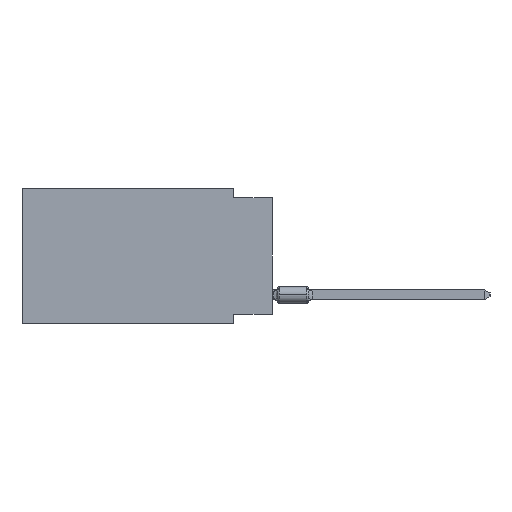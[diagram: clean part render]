
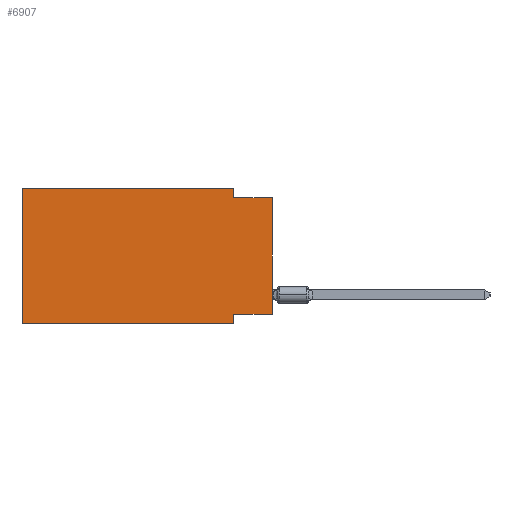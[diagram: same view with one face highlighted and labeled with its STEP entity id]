
A CAD part, left-side view. The second image highlights one B-rep face of the part: STEP entity #6907.
In plain terms, the highlighted planar face has unit normal (-1, 0, 0).
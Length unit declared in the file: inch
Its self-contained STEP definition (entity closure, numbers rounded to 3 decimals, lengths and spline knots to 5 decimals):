
#610 = VECTOR ( 'NONE', #41238, 39.37008 ) ;
#1041 = VECTOR ( 'NONE', #1689, 39.37008 ) ;
#1187 = VECTOR ( 'NONE', #8489, 39.37008 ) ;
#1689 = DIRECTION ( 'NONE',  ( 0., -1., 0. ) ) ;
#2277 = CARTESIAN_POINT ( 'NONE',  ( 0., 0.1, 0. ) ) ;
#2624 = CARTESIAN_POINT ( 'NONE',  ( 0., 0.1, -0.35 ) ) ;
#3584 = ORIENTED_EDGE ( 'NONE', *, *, #57239, .F. ) ;
#3718 = LINE ( 'NONE', #58554, #53860 ) ;
#4580 = VECTOR ( 'NONE', #31897, 39.37008 ) ;
#5265 = AXIS2_PLACEMENT_3D ( 'NONE', #47965, #54159, #21630 ) ;
#6539 = VECTOR ( 'NONE', #70454, 39.37008 ) ;
#6708 = EDGE_LOOP ( 'NONE', ( #24341, #24672, #17995, #44795, #29395, #54396, #44613, #3584 ) ) ;
#6907 = ADVANCED_FACE ( 'NONE', ( #42833 ), #60346, .F. ) ;
#7914 = VERTEX_POINT ( 'NONE', #2277 ) ;
#8489 = DIRECTION ( 'NONE',  ( 0., 0., -1. ) ) ;
#9325 = CARTESIAN_POINT ( 'NONE',  ( 0., 0.645, -0.35 ) ) ;
#17995 = ORIENTED_EDGE ( 'NONE', *, *, #40372, .F. ) ;
#19699 = LINE ( 'NONE', #24087, #38168 ) ;
#21630 = DIRECTION ( 'NONE',  ( 0., 0., -1. ) ) ;
#22252 = CARTESIAN_POINT ( 'NONE',  ( 0., 0.1, -0.325 ) ) ;
#22635 = DIRECTION ( 'NONE',  ( 0., 0., 1. ) ) ;
#22659 = VECTOR ( 'NONE', #22635, 39.37008 ) ;
#24087 = CARTESIAN_POINT ( 'NONE',  ( 0., 0.1, 0. ) ) ;
#24341 = ORIENTED_EDGE ( 'NONE', *, *, #68947, .T. ) ;
#24672 = ORIENTED_EDGE ( 'NONE', *, *, #59689, .F. ) ;
#24798 = CARTESIAN_POINT ( 'NONE',  ( 0., 0., 0. ) ) ;
#27245 = CARTESIAN_POINT ( 'NONE',  ( 0., 0., -0.025 ) ) ;
#29395 = ORIENTED_EDGE ( 'NONE', *, *, #30572, .F. ) ;
#30572 = EDGE_CURVE ( 'NONE', #43795, #34053, #61739, .T. ) ;
#30581 = LINE ( 'NONE', #52861, #1041 ) ;
#31017 = CARTESIAN_POINT ( 'NONE',  ( 0., 0., -0.325 ) ) ;
#31897 = DIRECTION ( 'NONE',  ( 0., -1., 0. ) ) ;
#33241 = CARTESIAN_POINT ( 'NONE',  ( 0., 0.645, 0. ) ) ;
#34053 = VERTEX_POINT ( 'NONE', #42239 ) ;
#34160 = VERTEX_POINT ( 'NONE', #27245 ) ;
#37383 = LINE ( 'NONE', #59661, #4580 ) ;
#38168 = VECTOR ( 'NONE', #47091, 39.37008 ) ;
#38562 = VERTEX_POINT ( 'NONE', #22252 ) ;
#40372 = EDGE_CURVE ( 'NONE', #7914, #53536, #19699, .T. ) ;
#41238 = DIRECTION ( 'NONE',  ( 0., 0., 1. ) ) ;
#42239 = CARTESIAN_POINT ( 'NONE',  ( 0., 0.645, 0. ) ) ;
#42833 = FACE_OUTER_BOUND ( 'NONE', #6708, .T. ) ;
#43795 = VERTEX_POINT ( 'NONE', #9325 ) ;
#44613 = ORIENTED_EDGE ( 'NONE', *, *, #59525, .F. ) ;
#44795 = ORIENTED_EDGE ( 'NONE', *, *, #47844, .F. ) ;
#46733 = LINE ( 'NONE', #24798, #610 ) ;
#47091 = DIRECTION ( 'NONE',  ( 0., 0., -1. ) ) ;
#47842 = CARTESIAN_POINT ( 'NONE',  ( 0., 0., -0.325 ) ) ;
#47844 = EDGE_CURVE ( 'NONE', #34053, #7914, #37383, .T. ) ;
#47965 = CARTESIAN_POINT ( 'NONE',  ( 0., 0.645, 0. ) ) ;
#50519 = EDGE_CURVE ( 'NONE', #43795, #62457, #3718, .T. ) ;
#52721 = LINE ( 'NONE', #2624, #1187 ) ;
#52861 = CARTESIAN_POINT ( 'NONE',  ( 0., 0., -0.025 ) ) ;
#53536 = VERTEX_POINT ( 'NONE', #54072 ) ;
#53860 = VECTOR ( 'NONE', #54154, 39.37008 ) ;
#54072 = CARTESIAN_POINT ( 'NONE',  ( 0., 0.1, -0.025 ) ) ;
#54154 = DIRECTION ( 'NONE',  ( 0., -1., 0. ) ) ;
#54159 = DIRECTION ( 'NONE',  ( 1., 0., 0. ) ) ;
#54396 = ORIENTED_EDGE ( 'NONE', *, *, #50519, .T. ) ;
#55930 = VERTEX_POINT ( 'NONE', #31017 ) ;
#57239 = EDGE_CURVE ( 'NONE', #55930, #38562, #58800, .T. ) ;
#58554 = CARTESIAN_POINT ( 'NONE',  ( 0., 0.645, -0.35 ) ) ;
#58800 = LINE ( 'NONE', #47842, #6539 ) ;
#59525 = EDGE_CURVE ( 'NONE', #38562, #62457, #52721, .T. ) ;
#59661 = CARTESIAN_POINT ( 'NONE',  ( 0., 0.645, 0. ) ) ;
#59689 = EDGE_CURVE ( 'NONE', #53536, #34160, #30581, .T. ) ;
#60346 = PLANE ( 'NONE',  #5265 ) ;
#61739 = LINE ( 'NONE', #33241, #22659 ) ;
#62457 = VERTEX_POINT ( 'NONE', #64987 ) ;
#64987 = CARTESIAN_POINT ( 'NONE',  ( 0., 0.1, -0.35 ) ) ;
#68947 = EDGE_CURVE ( 'NONE', #55930, #34160, #46733, .T. ) ;
#70454 = DIRECTION ( 'NONE',  ( 0., 1., 0. ) ) ;
